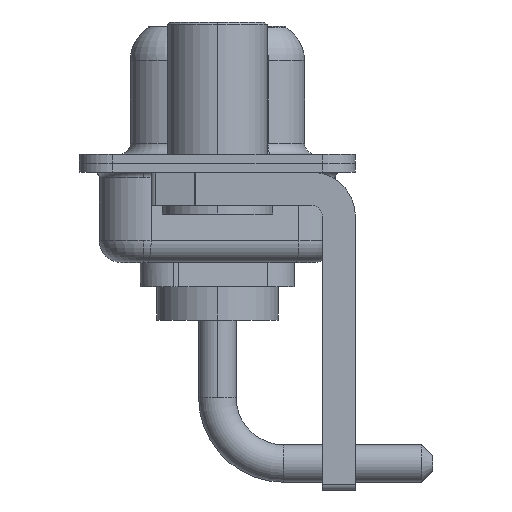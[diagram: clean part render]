
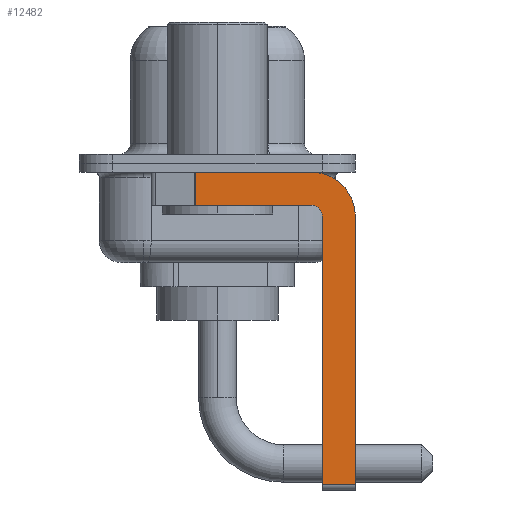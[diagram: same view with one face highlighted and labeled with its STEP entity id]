
A CAD part, left-side view. The second image highlights one B-rep face of the part: STEP entity #12482.
In plain terms, the highlighted planar face has unit normal (-1, 0, 0).
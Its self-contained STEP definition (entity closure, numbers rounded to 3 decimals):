
#202 = EDGE_CURVE ( 'NONE', #13739, #4983, #5845, .T. ) ;
#213 = CARTESIAN_POINT ( 'NONE',  ( -2.9, -4.75, -14.8 ) ) ;
#471 = CARTESIAN_POINT ( 'NONE',  ( -2.9, -6.25, -2.4 ) ) ;
#744 = DIRECTION ( 'NONE',  ( 0., 0., -1. ) ) ;
#1133 = VERTEX_POINT ( 'NONE', #1837 ) ;
#1135 = LINE ( 'NONE', #8160, #3025 ) ;
#1189 = EDGE_CURVE ( 'NONE', #14859, #13739, #1135, .T. ) ;
#1355 = DIRECTION ( 'NONE',  ( 0., 0., 1. ) ) ;
#1557 = VECTOR ( 'NONE', #744, 1000. ) ;
#1674 = LINE ( 'NONE', #11315, #1557 ) ;
#1837 = CARTESIAN_POINT ( 'NONE',  ( -2.9, -4.25, -1.9 ) ) ;
#2138 = DIRECTION ( 'NONE',  ( 0., -1., 0. ) ) ;
#3025 = VECTOR ( 'NONE', #2138, 1000. ) ;
#3193 = VERTEX_POINT ( 'NONE', #8889 ) ;
#3674 = EDGE_CURVE ( 'NONE', #4983, #9640, #1674, .T. ) ;
#4062 = CIRCLE ( 'NONE', #13153, 0.5 ) ;
#4426 = EDGE_CURVE ( 'NONE', #3193, #1133, #4062, .T. ) ;
#4488 = ORIENTED_EDGE ( 'NONE', *, *, #10064, .T. ) ;
#4561 = DIRECTION ( 'NONE',  ( 0., 1., 0. ) ) ;
#4633 = VERTEX_POINT ( 'NONE', #9680 ) ;
#4649 = ORIENTED_EDGE ( 'NONE', *, *, #11855, .F. ) ;
#4983 = VERTEX_POINT ( 'NONE', #471 ) ;
#5210 = CARTESIAN_POINT ( 'NONE',  ( -2.9, -4.25, -2.4 ) ) ;
#5576 = CARTESIAN_POINT ( 'NONE',  ( -2.9, -4.25, -2.4 ) ) ;
#5652 = VECTOR ( 'NONE', #4561, 1000. ) ;
#5657 = EDGE_CURVE ( 'NONE', #14859, #14503, #7626, .T. ) ;
#5845 = CIRCLE ( 'NONE', #6819, 2. ) ;
#5852 = DIRECTION ( 'NONE',  ( 0., -1., 0. ) ) ;
#5857 = CARTESIAN_POINT ( 'NONE',  ( -2.9, -4.25, -1.9 ) ) ;
#6126 = CARTESIAN_POINT ( 'NONE',  ( -2.9, 0.978, -1.9 ) ) ;
#6308 = DIRECTION ( 'NONE',  ( 0., 0., -1. ) ) ;
#6434 = VECTOR ( 'NONE', #6308, 1000. ) ;
#6550 = ORIENTED_EDGE ( 'NONE', *, *, #3674, .F. ) ;
#6795 = EDGE_CURVE ( 'NONE', #1133, #14503, #15026, .T. ) ;
#6819 = AXIS2_PLACEMENT_3D ( 'NONE', #5210, #11228, #7763 ) ;
#7208 = VECTOR ( 'NONE', #14113, 1000. ) ;
#7626 = LINE ( 'NONE', #12479, #6434 ) ;
#7763 = DIRECTION ( 'NONE',  ( 0., 0., -1. ) ) ;
#7901 = VECTOR ( 'NONE', #5852, 1000. ) ;
#8073 = CARTESIAN_POINT ( 'NONE',  ( -2.9, -4.25, -2.4 ) ) ;
#8126 = CARTESIAN_POINT ( 'NONE',  ( -2.9, 0.978, -0.4 ) ) ;
#8160 = CARTESIAN_POINT ( 'NONE',  ( -2.9, 3., -0.4 ) ) ;
#8435 = ORIENTED_EDGE ( 'NONE', *, *, #4426, .F. ) ;
#8889 = CARTESIAN_POINT ( 'NONE',  ( -2.9, -4.75, -2.4 ) ) ;
#9205 = DIRECTION ( 'NONE',  ( 1., 0., 0. ) ) ;
#9242 = ORIENTED_EDGE ( 'NONE', *, *, #202, .F. ) ;
#9287 = PLANE ( 'NONE',  #10676 ) ;
#9321 = EDGE_LOOP ( 'NONE', ( #9751, #9371, #13394, #8435, #4649, #4488, #6550, #9242 ) ) ;
#9371 = ORIENTED_EDGE ( 'NONE', *, *, #5657, .T. ) ;
#9408 = LINE ( 'NONE', #213, #7208 ) ;
#9640 = VERTEX_POINT ( 'NONE', #13908 ) ;
#9680 = CARTESIAN_POINT ( 'NONE',  ( -2.9, -4.75, -14.55 ) ) ;
#9751 = ORIENTED_EDGE ( 'NONE', *, *, #1189, .F. ) ;
#10064 = EDGE_CURVE ( 'NONE', #4633, #9640, #15098, .T. ) ;
#10473 = CARTESIAN_POINT ( 'NONE',  ( -2.9, -4.25, -0.4 ) ) ;
#10676 = AXIS2_PLACEMENT_3D ( 'NONE', #5576, #9205, #11445 ) ;
#11228 = DIRECTION ( 'NONE',  ( 1., 0., 0. ) ) ;
#11315 = CARTESIAN_POINT ( 'NONE',  ( -2.9, -6.25, -2.4 ) ) ;
#11445 = DIRECTION ( 'NONE',  ( 0., 0., -1. ) ) ;
#11855 = EDGE_CURVE ( 'NONE', #4633, #3193, #9408, .T. ) ;
#12479 = CARTESIAN_POINT ( 'NONE',  ( -2.9, 0.978, -1.9 ) ) ;
#12482 = ADVANCED_FACE ( 'NONE', ( #13902 ), #9287, .F. ) ;
#13153 = AXIS2_PLACEMENT_3D ( 'NONE', #8073, #14010, #1355 ) ;
#13394 = ORIENTED_EDGE ( 'NONE', *, *, #6795, .F. ) ;
#13739 = VERTEX_POINT ( 'NONE', #10473 ) ;
#13876 = CARTESIAN_POINT ( 'NONE',  ( -2.9, -4.25, -14.55 ) ) ;
#13902 = FACE_OUTER_BOUND ( 'NONE', #9321, .T. ) ;
#13908 = CARTESIAN_POINT ( 'NONE',  ( -2.9, -6.25, -14.55 ) ) ;
#14010 = DIRECTION ( 'NONE',  ( -1., 0., 0. ) ) ;
#14113 = DIRECTION ( 'NONE',  ( 0., 0., 1. ) ) ;
#14503 = VERTEX_POINT ( 'NONE', #6126 ) ;
#14859 = VERTEX_POINT ( 'NONE', #8126 ) ;
#15026 = LINE ( 'NONE', #5857, #5652 ) ;
#15098 = LINE ( 'NONE', #13876, #7901 ) ;
